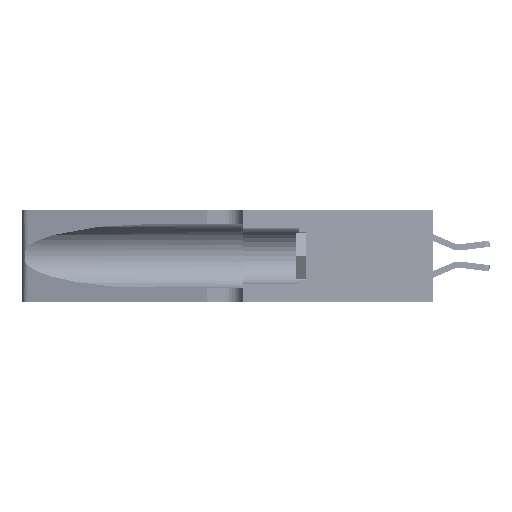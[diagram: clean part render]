
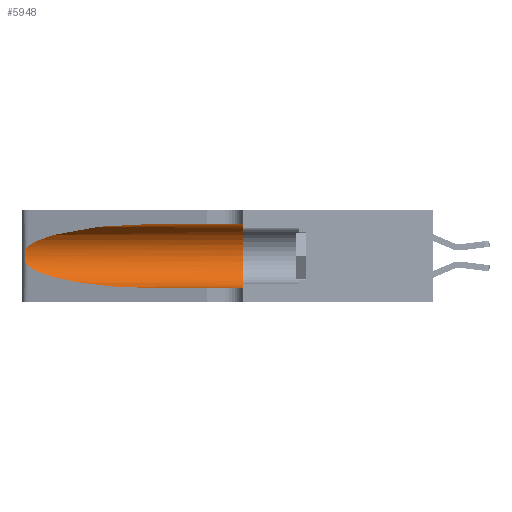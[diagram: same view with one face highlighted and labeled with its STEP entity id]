
A CAD part, left-side view. The second image highlights one B-rep face of the part: STEP entity #5948.
In plain terms, the highlighted cylindrical face has radius 3.308 mm (diameter 6.617 mm), a partial arc.
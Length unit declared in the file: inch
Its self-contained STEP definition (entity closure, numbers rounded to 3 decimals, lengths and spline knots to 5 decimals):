
#234 = CARTESIAN_POINT ( 'NONE',  ( 0.26075, 1.23896, 0.19203 ) ) ;
#3071 = ORIENTED_EDGE ( 'NONE', *, *, #32576, .F. ) ;
#3733 = CARTESIAN_POINT ( 'NONE',  ( 0.26017, 1.23833, 0.17102 ) ) ;
#4005 = EDGE_CURVE ( 'NONE', #37395, #12721, #29438, .T. ) ;
#4464 = CARTESIAN_POINT ( 'NONE',  ( 0.1305, 0.35, 0.31525 ) ) ;
#5727 = ORIENTED_EDGE ( 'NONE', *, *, #10367, .T. ) ;
#5948 = ADVANCED_FACE ( 'NONE', ( #6741 ), #23017, .F. ) ;
#6563 = CARTESIAN_POINT ( 'NONE',  ( 0.2373, 1.15595, 0.08982 ) ) ;
#6741 = FACE_OUTER_BOUND ( 'NONE', #26951, .T. ) ;
#7213 = CARTESIAN_POINT ( 'NONE',  ( 0.25789, 1.23486, 0.15765 ) ) ;
#9008 = ORIENTED_EDGE ( 'NONE', *, *, #21233, .T. ) ;
#10105 = CARTESIAN_POINT ( 'NONE',  ( 0.25487, 1.22718, 0.22369 ) ) ;
#10315 = EDGE_CURVE ( 'NONE', #43734, #31534, #13942, .T. ) ;
#10367 = EDGE_CURVE ( 'NONE', #14633, #43734, #23126, .T. ) ;
#10580 = CARTESIAN_POINT ( 'NONE',  ( 0.25487, 1.22718, 0.22369 ) ) ;
#10729 = CARTESIAN_POINT ( 'NONE',  ( 0.25555, 1.22993, 0.14849 ) ) ;
#11749 =( BOUNDED_CURVE ( )  B_SPLINE_CURVE ( 3, ( #30497, #37406, #16814, #40904 ),
 .UNSPECIFIED., .F., .F. ) 
 B_SPLINE_CURVE_WITH_KNOTS ( ( 4, 4 ),
 ( 1.5708, 2.84003 ),
 .UNSPECIFIED. ) 
 CURVE ( )  GEOMETRIC_REPRESENTATION_ITEM ( )  RATIONAL_B_SPLINE_CURVE ( ( 1., 0.87, 0.87, 1. ) ) 
 REPRESENTATION_ITEM ( '' )  );
#11775 = VECTOR ( 'NONE', #16595, 39.37008 ) ;
#11941 = DIRECTION ( 'NONE',  ( 0., -1., 0. ) ) ;
#12721 = VERTEX_POINT ( 'NONE', #4464 ) ;
#13942 = LINE ( 'NONE', #33744, #11775 ) ;
#14063 = CARTESIAN_POINT ( 'NONE',  ( 0.25555, 1.22994, 0.2215 ) ) ;
#14335 = AXIS2_PLACEMENT_3D ( 'NONE', #15250, #11941, #15407 ) ;
#14633 = VERTEX_POINT ( 'NONE', #21762 ) ;
#15250 = CARTESIAN_POINT ( 'NONE',  ( 0.1305, 1.61858, 0.185 ) ) ;
#15407 = DIRECTION ( 'NONE',  ( 0., 0., -1. ) ) ;
#16595 = DIRECTION ( 'NONE',  ( 0., -1., 0. ) ) ;
#16814 = CARTESIAN_POINT ( 'NONE',  ( 0.2373, 1.15595, 0.28018 ) ) ;
#17540 = CARTESIAN_POINT ( 'NONE',  ( 0.25787, 1.23484, 0.2124 ) ) ;
#17588 = CARTESIAN_POINT ( 'NONE',  ( 0.1305, 0.35, 0.185 ) ) ;
#19129 = AXIS2_PLACEMENT_3D ( 'NONE', #17588, #41633, #21051 ) ;
#21005 = CARTESIAN_POINT ( 'NONE',  ( 0.26018, 1.23835, 0.19895 ) ) ;
#21051 = DIRECTION ( 'NONE',  ( 0., 0., 1. ) ) ;
#21233 = EDGE_CURVE ( 'NONE', #42944, #14633, #35723, .T. ) ;
#21762 = CARTESIAN_POINT ( 'NONE',  ( 0.25487, 1.22718, 0.14631 ) ) ;
#23017 = CYLINDRICAL_SURFACE ( 'NONE', #14335, 0.13025 ) ;
#23126 =( BOUNDED_CURVE ( )  B_SPLINE_CURVE ( 3, ( #30727, #6563, #27295, #34179 ),
 .UNSPECIFIED., .F., .F. ) 
 B_SPLINE_CURVE_WITH_KNOTS ( ( 4, 4 ),
 ( 3.44316, 4.71239 ),
 .UNSPECIFIED. ) 
 CURVE ( )  GEOMETRIC_REPRESENTATION_ITEM ( )  RATIONAL_B_SPLINE_CURVE ( ( 1., 0.87, 0.87, 1. ) ) 
 REPRESENTATION_ITEM ( '' )  );
#24214 = EDGE_CURVE ( 'NONE', #37395, #42944, #11749, .T. ) ;
#24477 = CARTESIAN_POINT ( 'NONE',  ( 0.26075, 1.23896, 0.178 ) ) ;
#25217 = ORIENTED_EDGE ( 'NONE', *, *, #4005, .F. ) ;
#26951 = EDGE_LOOP ( 'NONE', ( #44357, #9008, #5727, #35483, #3071, #25217 ) ) ;
#27295 = CARTESIAN_POINT ( 'NONE',  ( 0.18966, 0.96281, 0.05475 ) ) ;
#27932 = CARTESIAN_POINT ( 'NONE',  ( 0.25856, 1.23593, 0.16098 ) ) ;
#29438 = LINE ( 'NONE', #44114, #36416 ) ;
#30497 = CARTESIAN_POINT ( 'NONE',  ( 0.1305, 0.72297, 0.31525 ) ) ;
#30727 = CARTESIAN_POINT ( 'NONE',  ( 0.25487, 1.22718, 0.14631 ) ) ;
#30761 = CARTESIAN_POINT ( 'NONE',  ( 0.1305, 0.72297, 0.31525 ) ) ;
#31373 = CARTESIAN_POINT ( 'NONE',  ( 0.25639, 1.23186, 0.15144 ) ) ;
#31534 = VERTEX_POINT ( 'NONE', #32391 ) ;
#32391 = CARTESIAN_POINT ( 'NONE',  ( 0.1305, 0.35, 0.05475 ) ) ;
#32576 = EDGE_CURVE ( 'NONE', #12721, #31534, #35202, .T. ) ;
#33744 = CARTESIAN_POINT ( 'NONE',  ( 0.1305, 1.61858, 0.05475 ) ) ;
#34179 = CARTESIAN_POINT ( 'NONE',  ( 0.1305, 0.72297, 0.05475 ) ) ;
#34810 = CARTESIAN_POINT ( 'NONE',  ( 0.25487, 1.22718, 0.14631 ) ) ;
#35202 = CIRCLE ( 'NONE', #19129, 0.13025 ) ;
#35483 = ORIENTED_EDGE ( 'NONE', *, *, #10315, .T. ) ;
#35723 = B_SPLINE_CURVE_WITH_KNOTS ( 'NONE', 3,
 ( #10580, #14063, #38124, #17540, #41598, #21005, #234, #24477, #3733, #27932, #7213, #31373, #10729, #34810 ),
 .UNSPECIFIED., .F., .F.,
 ( 4, 2, 2, 2, 2, 2, 4 ),
 ( 0., 0.00027, 0.00053, 0.00107, 0.0016, 0.00187, 0.00214 ),
 .UNSPECIFIED. ) ;
#36416 = VECTOR ( 'NONE', #40825, 39.37008 ) ;
#37395 = VERTEX_POINT ( 'NONE', #30761 ) ;
#37406 = CARTESIAN_POINT ( 'NONE',  ( 0.18966, 0.96281, 0.31525 ) ) ;
#38124 = CARTESIAN_POINT ( 'NONE',  ( 0.25639, 1.23184, 0.21858 ) ) ;
#40825 = DIRECTION ( 'NONE',  ( 0., -1., 0. ) ) ;
#40904 = CARTESIAN_POINT ( 'NONE',  ( 0.25487, 1.22718, 0.22369 ) ) ;
#41598 = CARTESIAN_POINT ( 'NONE',  ( 0.25854, 1.2359, 0.20912 ) ) ;
#41633 = DIRECTION ( 'NONE',  ( 0., 1., 0. ) ) ;
#41645 = CARTESIAN_POINT ( 'NONE',  ( 0.1305, 0.72297, 0.05475 ) ) ;
#42944 = VERTEX_POINT ( 'NONE', #10105 ) ;
#43734 = VERTEX_POINT ( 'NONE', #41645 ) ;
#44114 = CARTESIAN_POINT ( 'NONE',  ( 0.1305, 1.61858, 0.31525 ) ) ;
#44357 = ORIENTED_EDGE ( 'NONE', *, *, #24214, .T. ) ;
